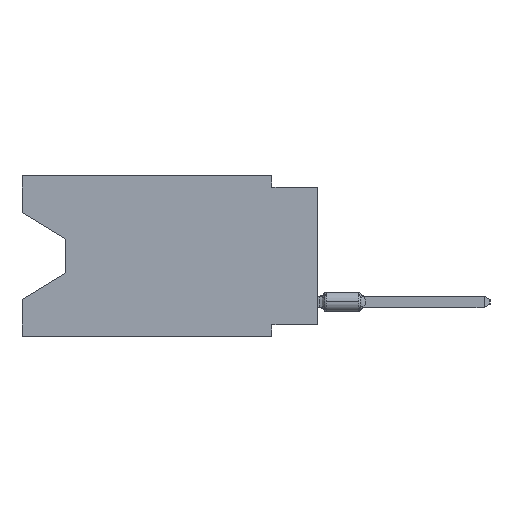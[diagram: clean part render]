
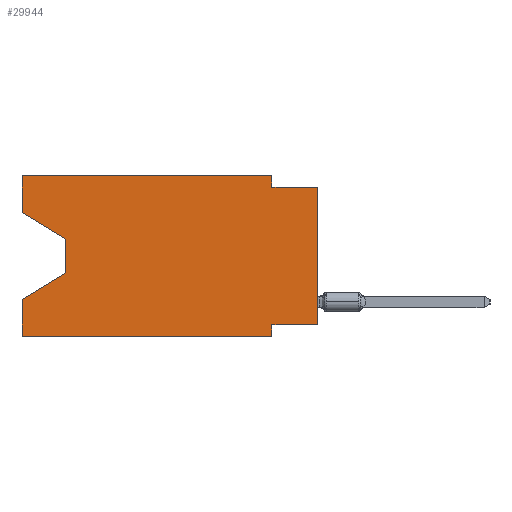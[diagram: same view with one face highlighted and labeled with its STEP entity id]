
A CAD part, left-side view. The second image highlights one B-rep face of the part: STEP entity #29944.
In plain terms, the highlighted planar face has unit normal (-1, 0, 0).
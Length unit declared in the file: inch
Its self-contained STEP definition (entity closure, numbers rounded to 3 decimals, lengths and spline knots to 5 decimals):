
#175 = ORIENTED_EDGE ( 'NONE', *, *, #20613, .F. ) ;
#339 = VERTEX_POINT ( 'NONE', #32168 ) ;
#638 = LINE ( 'NONE', #28819, #30809 ) ;
#896 = EDGE_CURVE ( 'NONE', #23127, #24977, #27203, .T. ) ;
#1205 = ORIENTED_EDGE ( 'NONE', *, *, #33406, .F. ) ;
#1346 = VERTEX_POINT ( 'NONE', #26789 ) ;
#1431 = CARTESIAN_POINT ( 'NONE',  ( 0., 0., -0.025 ) ) ;
#2289 = VECTOR ( 'NONE', #16964, 39.37008 ) ;
#2505 = DIRECTION ( 'NONE',  ( 0., -0.855, -0.519 ) ) ;
#3204 = AXIS2_PLACEMENT_3D ( 'NONE', #23166, #17959, #31880 ) ;
#3672 = PLANE ( 'NONE',  #3204 ) ;
#4535 = EDGE_CURVE ( 'NONE', #30178, #36214, #11637, .T. ) ;
#5328 = DIRECTION ( 'NONE',  ( 0., 0.855, -0.519 ) ) ;
#5696 = LINE ( 'NONE', #30370, #13538 ) ;
#5719 = DIRECTION ( 'NONE',  ( 0., 1., 0. ) ) ;
#6013 = VERTEX_POINT ( 'NONE', #25347 ) ;
#6455 = EDGE_CURVE ( 'NONE', #29000, #8534, #9225, .T. ) ;
#7652 = ORIENTED_EDGE ( 'NONE', *, *, #30683, .T. ) ;
#8534 = VERTEX_POINT ( 'NONE', #15310 ) ;
#8716 = EDGE_CURVE ( 'NONE', #30178, #339, #22723, .T. ) ;
#9225 = LINE ( 'NONE', #31483, #13304 ) ;
#9275 = ORIENTED_EDGE ( 'NONE', *, *, #14106, .T. ) ;
#9388 = LINE ( 'NONE', #11985, #10085 ) ;
#9949 = VECTOR ( 'NONE', #2505, 39.37008 ) ;
#10085 = VECTOR ( 'NONE', #31659, 39.37008 ) ;
#10401 = CARTESIAN_POINT ( 'NONE',  ( 0., 0., -0.025 ) ) ;
#10725 = CARTESIAN_POINT ( 'NONE',  ( 0., 0., -0.325 ) ) ;
#11275 = DIRECTION ( 'NONE',  ( 0., 0., 1. ) ) ;
#11412 = VECTOR ( 'NONE', #5719, 39.37008 ) ;
#11421 = VECTOR ( 'NONE', #11275, 39.37008 ) ;
#11637 = LINE ( 'NONE', #17203, #11421 ) ;
#11985 = CARTESIAN_POINT ( 'NONE',  ( 0., 0.55, -0.138 ) ) ;
#12132 = DIRECTION ( 'NONE',  ( 0., 0., -1. ) ) ;
#12551 = LINE ( 'NONE', #34280, #26531 ) ;
#12824 = ORIENTED_EDGE ( 'NONE', *, *, #30417, .T. ) ;
#13099 = DIRECTION ( 'NONE',  ( 0., -1., 0. ) ) ;
#13304 = VECTOR ( 'NONE', #31674, 39.37008 ) ;
#13538 = VECTOR ( 'NONE', #5328, 39.37008 ) ;
#14106 = EDGE_CURVE ( 'NONE', #20381, #1346, #5696, .T. ) ;
#14975 = DIRECTION ( 'NONE',  ( 0., -1., 0. ) ) ;
#15310 = CARTESIAN_POINT ( 'NONE',  ( 0., 0.1, -0.35 ) ) ;
#16964 = DIRECTION ( 'NONE',  ( 0., 0., 1. ) ) ;
#17148 = LINE ( 'NONE', #22539, #2289 ) ;
#17203 = CARTESIAN_POINT ( 'NONE',  ( 0., 0.645, 0. ) ) ;
#17525 = CARTESIAN_POINT ( 'NONE',  ( 0., 0.645, -0.35 ) ) ;
#17959 = DIRECTION ( 'NONE',  ( 1., 0., 0. ) ) ;
#18245 = EDGE_CURVE ( 'NONE', #29000, #1346, #25089, .T. ) ;
#18420 = CARTESIAN_POINT ( 'NONE',  ( 0., 0.1, -0.325 ) ) ;
#18859 = ORIENTED_EDGE ( 'NONE', *, *, #18245, .F. ) ;
#19884 = VECTOR ( 'NONE', #13099, 39.37008 ) ;
#20381 = VERTEX_POINT ( 'NONE', #31447 ) ;
#20613 = EDGE_CURVE ( 'NONE', #6013, #23127, #12551, .T. ) ;
#20729 = CARTESIAN_POINT ( 'NONE',  ( 0., 0.645, 0. ) ) ;
#21326 = ORIENTED_EDGE ( 'NONE', *, *, #6455, .T. ) ;
#21595 = CARTESIAN_POINT ( 'NONE',  ( 0., 0.1, -0.025 ) ) ;
#21674 = VECTOR ( 'NONE', #36422, 39.37008 ) ;
#22017 = ORIENTED_EDGE ( 'NONE', *, *, #896, .F. ) ;
#22188 = CARTESIAN_POINT ( 'NONE',  ( 0., 0.645, -0.08025 ) ) ;
#22539 = CARTESIAN_POINT ( 'NONE',  ( 0., 0., 0. ) ) ;
#22723 = LINE ( 'NONE', #22188, #9949 ) ;
#23127 = VERTEX_POINT ( 'NONE', #21595 ) ;
#23166 = CARTESIAN_POINT ( 'NONE',  ( 0., 0.645, 0. ) ) ;
#24940 = VECTOR ( 'NONE', #14975, 39.37008 ) ;
#24977 = VERTEX_POINT ( 'NONE', #10401 ) ;
#25089 = LINE ( 'NONE', #31551, #21674 ) ;
#25347 = CARTESIAN_POINT ( 'NONE',  ( 0., 0.1, 0. ) ) ;
#25748 = CARTESIAN_POINT ( 'NONE',  ( 0., 0.645, 0. ) ) ;
#26531 = VECTOR ( 'NONE', #31495, 39.37008 ) ;
#26560 = VERTEX_POINT ( 'NONE', #34541 ) ;
#26789 = CARTESIAN_POINT ( 'NONE',  ( 0., 0.645, -0.26975 ) ) ;
#27203 = LINE ( 'NONE', #1431, #19884 ) ;
#27414 = VERTEX_POINT ( 'NONE', #18420 ) ;
#27679 = ORIENTED_EDGE ( 'NONE', *, *, #28518, .F. ) ;
#28518 = EDGE_CURVE ( 'NONE', #26560, #27414, #36158, .T. ) ;
#28819 = CARTESIAN_POINT ( 'NONE',  ( 0., 0.1, -0.35 ) ) ;
#29000 = VERTEX_POINT ( 'NONE', #17525 ) ;
#29944 = ADVANCED_FACE ( 'NONE', ( #33760 ), #3672, .F. ) ;
#30178 = VERTEX_POINT ( 'NONE', #35583 ) ;
#30201 = ORIENTED_EDGE ( 'NONE', *, *, #31975, .F. ) ;
#30370 = CARTESIAN_POINT ( 'NONE',  ( 0., 0.55, -0.212 ) ) ;
#30417 = EDGE_CURVE ( 'NONE', #339, #20381, #9388, .T. ) ;
#30683 = EDGE_CURVE ( 'NONE', #26560, #24977, #17148, .T. ) ;
#30809 = VECTOR ( 'NONE', #12132, 39.37008 ) ;
#31447 = CARTESIAN_POINT ( 'NONE',  ( 0., 0.55, -0.212 ) ) ;
#31483 = CARTESIAN_POINT ( 'NONE',  ( 0., 0.645, -0.35 ) ) ;
#31495 = DIRECTION ( 'NONE',  ( 0., 0., -1. ) ) ;
#31551 = CARTESIAN_POINT ( 'NONE',  ( 0., 0.645, 0. ) ) ;
#31659 = DIRECTION ( 'NONE',  ( 0., 0., -1. ) ) ;
#31674 = DIRECTION ( 'NONE',  ( 0., -1., 0. ) ) ;
#31880 = DIRECTION ( 'NONE',  ( 0., 0., -1. ) ) ;
#31975 = EDGE_CURVE ( 'NONE', #27414, #8534, #638, .T. ) ;
#32017 = ORIENTED_EDGE ( 'NONE', *, *, #4535, .F. ) ;
#32168 = CARTESIAN_POINT ( 'NONE',  ( 0., 0.55, -0.138 ) ) ;
#32984 = ORIENTED_EDGE ( 'NONE', *, *, #8716, .T. ) ;
#33406 = EDGE_CURVE ( 'NONE', #36214, #6013, #35716, .T. ) ;
#33482 = EDGE_LOOP ( 'NONE', ( #32984, #12824, #9275, #18859, #21326, #30201, #27679, #7652, #22017, #175, #1205, #32017 ) ) ;
#33760 = FACE_OUTER_BOUND ( 'NONE', #33482, .T. ) ;
#34280 = CARTESIAN_POINT ( 'NONE',  ( 0., 0.1, 0. ) ) ;
#34541 = CARTESIAN_POINT ( 'NONE',  ( 0., 0., -0.325 ) ) ;
#35583 = CARTESIAN_POINT ( 'NONE',  ( 0., 0.645, -0.08025 ) ) ;
#35716 = LINE ( 'NONE', #20729, #24940 ) ;
#36158 = LINE ( 'NONE', #10725, #11412 ) ;
#36214 = VERTEX_POINT ( 'NONE', #25748 ) ;
#36422 = DIRECTION ( 'NONE',  ( 0., 0., 1. ) ) ;
